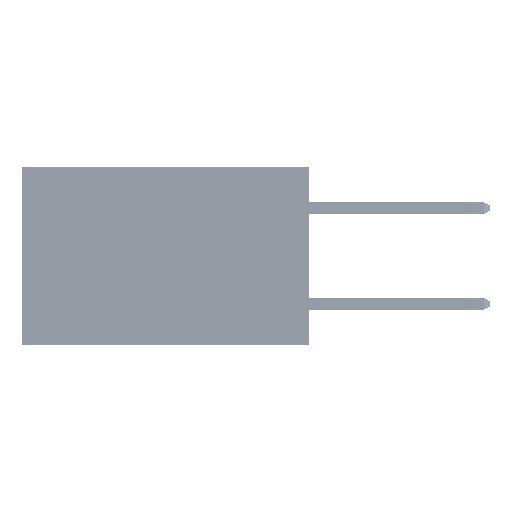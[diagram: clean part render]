
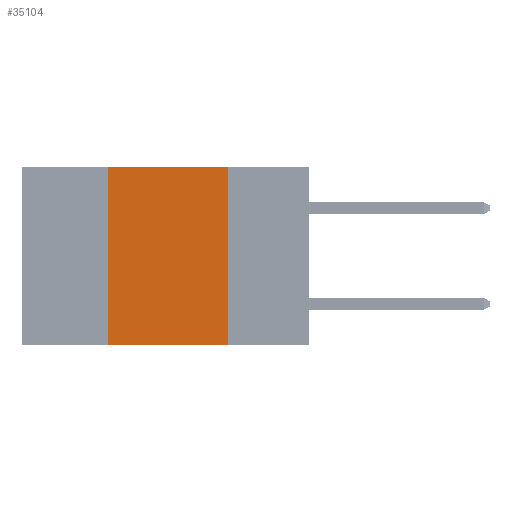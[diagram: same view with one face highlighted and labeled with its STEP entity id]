
A CAD part, left-side view. The second image highlights one B-rep face of the part: STEP entity #35104.
In plain terms, the highlighted planar face has unit normal (-1, 0, 0).
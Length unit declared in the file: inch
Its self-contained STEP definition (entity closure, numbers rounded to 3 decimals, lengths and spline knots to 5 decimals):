
#402 = VERTEX_POINT ( 'NONE', #10248 ) ;
#2637 = CARTESIAN_POINT ( 'NONE',  ( 0., 0.6, 0. ) ) ;
#4864 = VERTEX_POINT ( 'NONE', #52320 ) ;
#5275 = VECTOR ( 'NONE', #43556, 39.37008 ) ;
#6709 = DIRECTION ( 'NONE',  ( 1., 0., 0. ) ) ;
#6809 = LINE ( 'NONE', #22172, #27730 ) ;
#9303 = DIRECTION ( 'NONE',  ( 0., -1., 0. ) ) ;
#10248 = CARTESIAN_POINT ( 'NONE',  ( 0., 0.42, -0.37 ) ) ;
#11588 = ORIENTED_EDGE ( 'NONE', *, *, #39857, .F. ) ;
#13021 = VECTOR ( 'NONE', #9303, 39.37008 ) ;
#13212 = EDGE_CURVE ( 'NONE', #402, #26445, #26866, .T. ) ;
#19984 = DIRECTION ( 'NONE',  ( 0., 0., -1. ) ) ;
#21921 = AXIS2_PLACEMENT_3D ( 'NONE', #2637, #6709, #19984 ) ;
#22172 = CARTESIAN_POINT ( 'NONE',  ( 0., 0.6, -0.37 ) ) ;
#23395 = ORIENTED_EDGE ( 'NONE', *, *, #29109, .T. ) ;
#24468 = DIRECTION ( 'NONE',  ( 0., 0., -1. ) ) ;
#25184 = FACE_OUTER_BOUND ( 'NONE', #25919, .T. ) ;
#25302 = VECTOR ( 'NONE', #24468, 39.37008 ) ;
#25919 = EDGE_LOOP ( 'NONE', ( #11588, #26711, #47237, #23395 ) ) ;
#26445 = VERTEX_POINT ( 'NONE', #47727 ) ;
#26711 = ORIENTED_EDGE ( 'NONE', *, *, #52173, .F. ) ;
#26866 = LINE ( 'NONE', #35935, #5275 ) ;
#27702 = VERTEX_POINT ( 'NONE', #28597 ) ;
#27730 = VECTOR ( 'NONE', #33562, 39.37008 ) ;
#28597 = CARTESIAN_POINT ( 'NONE',  ( 0., 0.17, 0. ) ) ;
#29109 = EDGE_CURVE ( 'NONE', #402, #4864, #6809, .T. ) ;
#31531 = PLANE ( 'NONE',  #21921 ) ;
#33562 = DIRECTION ( 'NONE',  ( 0., -1., 0. ) ) ;
#35104 = ADVANCED_FACE ( 'NONE', ( #25184 ), #31531, .F. ) ;
#35935 = CARTESIAN_POINT ( 'NONE',  ( 0., 0.42, 0. ) ) ;
#37159 = LINE ( 'NONE', #41588, #13021 ) ;
#39857 = EDGE_CURVE ( 'NONE', #27702, #4864, #41814, .T. ) ;
#41588 = CARTESIAN_POINT ( 'NONE',  ( 0., 0.6, 0. ) ) ;
#41814 = LINE ( 'NONE', #44862, #25302 ) ;
#43556 = DIRECTION ( 'NONE',  ( 0., 0., 1. ) ) ;
#44862 = CARTESIAN_POINT ( 'NONE',  ( 0., 0.17, 0. ) ) ;
#47237 = ORIENTED_EDGE ( 'NONE', *, *, #13212, .F. ) ;
#47727 = CARTESIAN_POINT ( 'NONE',  ( 0., 0.42, 0. ) ) ;
#52173 = EDGE_CURVE ( 'NONE', #26445, #27702, #37159, .T. ) ;
#52320 = CARTESIAN_POINT ( 'NONE',  ( 0., 0.17, -0.37 ) ) ;
